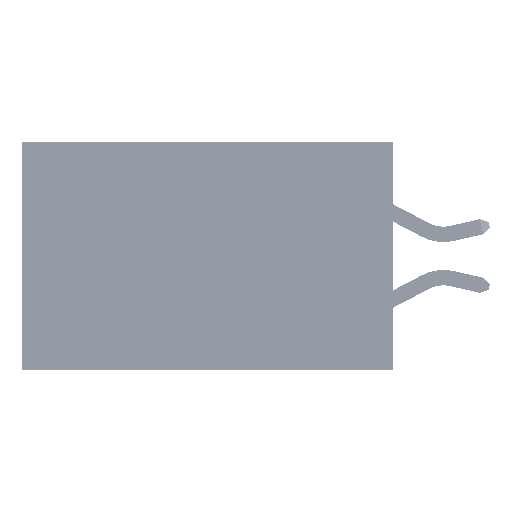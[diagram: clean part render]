
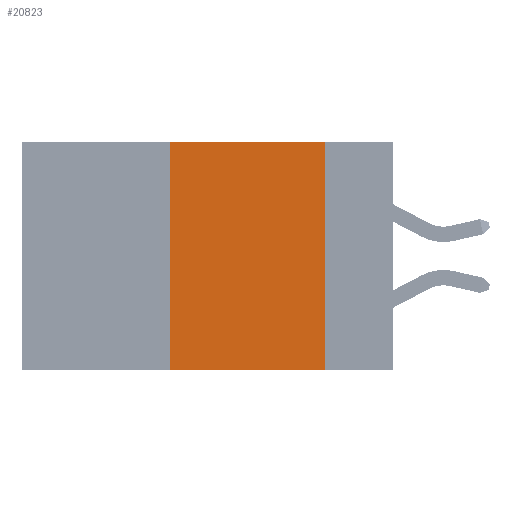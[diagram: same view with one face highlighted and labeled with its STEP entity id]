
A CAD part, left-side view. The second image highlights one B-rep face of the part: STEP entity #20823.
In plain terms, the highlighted planar face has unit normal (-1, 0, 0).
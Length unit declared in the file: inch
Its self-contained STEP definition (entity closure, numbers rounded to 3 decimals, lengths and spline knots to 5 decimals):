
#4345 = VECTOR ( 'NONE', #41272, 39.37008 ) ;
#6792 = DIRECTION ( 'NONE',  ( 0., 0., -1. ) ) ;
#10565 = CARTESIAN_POINT ( 'NONE',  ( 0., 0.11, -0.37 ) ) ;
#11626 = CARTESIAN_POINT ( 'NONE',  ( 0., 0.6, 0. ) ) ;
#12934 = LINE ( 'NONE', #17548, #4345 ) ;
#13279 = DIRECTION ( 'NONE',  ( 0., 0., 1. ) ) ;
#13626 = VECTOR ( 'NONE', #13279, 39.37008 ) ;
#15908 = FACE_OUTER_BOUND ( 'NONE', #20231, .T. ) ;
#16524 = CARTESIAN_POINT ( 'NONE',  ( 0., 0.36, 0. ) ) ;
#17548 = CARTESIAN_POINT ( 'NONE',  ( 0., 0.6, -0.37 ) ) ;
#18618 = EDGE_CURVE ( 'NONE', #40893, #31512, #12934, .T. ) ;
#18640 = CARTESIAN_POINT ( 'NONE',  ( 0., 0.11, 0. ) ) ;
#20231 = EDGE_LOOP ( 'NONE', ( #38034, #50419, #26210, #29172 ) ) ;
#20739 = LINE ( 'NONE', #50079, #39311 ) ;
#20823 = ADVANCED_FACE ( 'NONE', ( #15908 ), #47569, .F. ) ;
#22019 = AXIS2_PLACEMENT_3D ( 'NONE', #11626, #31538, #23964 ) ;
#22825 = CARTESIAN_POINT ( 'NONE',  ( 0., 0.36, -0.37 ) ) ;
#23488 = LINE ( 'NONE', #16524, #13626 ) ;
#23964 = DIRECTION ( 'NONE',  ( 0., 0., -1. ) ) ;
#26210 = ORIENTED_EDGE ( 'NONE', *, *, #41219, .F. ) ;
#29172 = ORIENTED_EDGE ( 'NONE', *, *, #18618, .T. ) ;
#29813 = CARTESIAN_POINT ( 'NONE',  ( 0., 0.11, 0. ) ) ;
#31512 = VERTEX_POINT ( 'NONE', #10565 ) ;
#31538 = DIRECTION ( 'NONE',  ( 1., 0., 0. ) ) ;
#33769 = EDGE_CURVE ( 'NONE', #34548, #47463, #20739, .T. ) ;
#34548 = VERTEX_POINT ( 'NONE', #42780 ) ;
#36153 = LINE ( 'NONE', #29813, #43621 ) ;
#38034 = ORIENTED_EDGE ( 'NONE', *, *, #43998, .F. ) ;
#39311 = VECTOR ( 'NONE', #42488, 39.37008 ) ;
#40893 = VERTEX_POINT ( 'NONE', #22825 ) ;
#41219 = EDGE_CURVE ( 'NONE', #40893, #34548, #23488, .T. ) ;
#41272 = DIRECTION ( 'NONE',  ( 0., -1., 0. ) ) ;
#42488 = DIRECTION ( 'NONE',  ( 0., -1., 0. ) ) ;
#42780 = CARTESIAN_POINT ( 'NONE',  ( 0., 0.36, 0. ) ) ;
#43621 = VECTOR ( 'NONE', #6792, 39.37008 ) ;
#43998 = EDGE_CURVE ( 'NONE', #47463, #31512, #36153, .T. ) ;
#47463 = VERTEX_POINT ( 'NONE', #18640 ) ;
#47569 = PLANE ( 'NONE',  #22019 ) ;
#50079 = CARTESIAN_POINT ( 'NONE',  ( 0., 0.6, 0. ) ) ;
#50419 = ORIENTED_EDGE ( 'NONE', *, *, #33769, .F. ) ;
